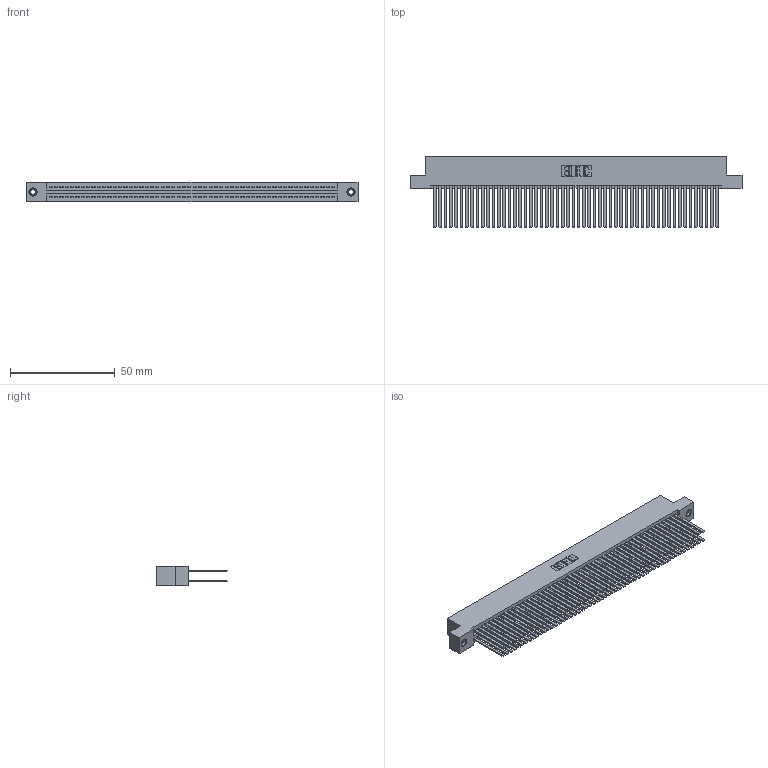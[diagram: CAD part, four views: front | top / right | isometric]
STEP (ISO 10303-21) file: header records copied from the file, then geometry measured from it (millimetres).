
FILE_DESCRIPTION (( 'STEP AP203' ), '1' );
FILE_NAME ('345-108-544-208.STEP', '2019-11-04T13:46:19', ( '' ), ( '' ), 'SwSTEP 2.0', 'SolidWorks 2016', '' );
FILE_SCHEMA (( 'CONFIG_CONTROL_DESIGN' ));
Length unit declared in the file: inch
Products named in the file (4): 345-292-001_345-293-144; 345-250-001_345-250-003-102; 345 Part_Flush Mounting Lugs - 0.156 Dia-TI; 345-108-544-208
Assembly tree (111 placements, depth 2):
  345-108-544-208
    345 Part_Flush Mounting Lugs - 0.156 Dia-TI
    345-292-001_345-293-144  x108
    345-250-001_345-250-003-102  x2
Bounding box: 158.37 x 33.96 x 9.4 mm (x, y, z)
Volume: 17003 mm3; surface area: 29816.4 mm2
Topology: 111 solids, 111 shells, 4938 faces, 14625 edges, 9598 vertices
Faces by surface type: plane 3244, cylinder 1678, cone 12, torus 4
Entity records: 41756 total; most frequent: CARTESIAN_POINT 6967, ORIENTED_EDGE 6894, DIRECTION 6153, EDGE_CURVE 3447, LINE 3083, VECTOR 3083, VERTEX_POINT 2292, AXIS2_PLACEMENT_3D 1535
